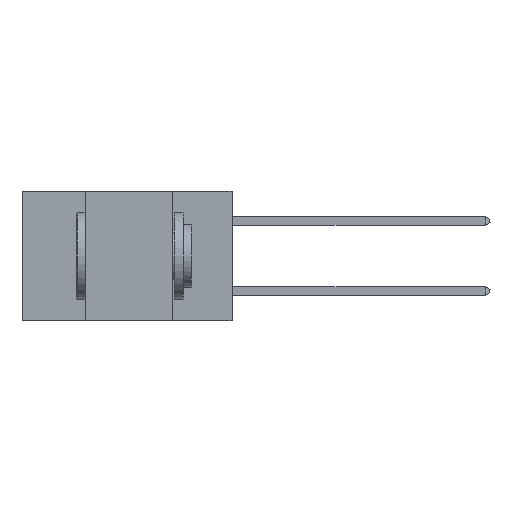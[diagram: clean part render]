
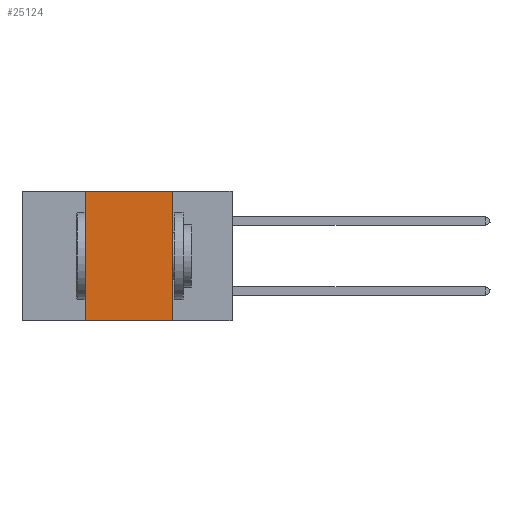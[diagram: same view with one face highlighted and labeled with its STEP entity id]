
A CAD part, left-side view. The second image highlights one B-rep face of the part: STEP entity #25124.
In plain terms, the highlighted planar face has unit normal (-1, 0, 0).
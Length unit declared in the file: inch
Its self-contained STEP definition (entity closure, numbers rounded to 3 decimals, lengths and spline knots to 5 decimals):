
#597 = CARTESIAN_POINT ( 'NONE',  ( 0., 0.42, -0.37 ) ) ;
#2726 = EDGE_CURVE ( 'NONE', #23165, #25789, #34216, .T. ) ;
#4073 = VERTEX_POINT ( 'NONE', #22299 ) ;
#4488 = CARTESIAN_POINT ( 'NONE',  ( 0., 0.6, 0. ) ) ;
#5153 = ORIENTED_EDGE ( 'NONE', *, *, #2726, .F. ) ;
#6057 = ORIENTED_EDGE ( 'NONE', *, *, #22233, .F. ) ;
#7336 = FACE_OUTER_BOUND ( 'NONE', #36327, .T. ) ;
#9321 = PLANE ( 'NONE',  #26371 ) ;
#10691 = VECTOR ( 'NONE', #11193, 39.37008 ) ;
#10835 = CARTESIAN_POINT ( 'NONE',  ( 0., 0.17, 0. ) ) ;
#11193 = DIRECTION ( 'NONE',  ( 0., 0., -1. ) ) ;
#12261 = CARTESIAN_POINT ( 'NONE',  ( 0., 0.17, -0.37 ) ) ;
#15567 = VECTOR ( 'NONE', #27453, 39.37008 ) ;
#17461 = VECTOR ( 'NONE', #36445, 39.37008 ) ;
#17555 = LINE ( 'NONE', #18975, #31771 ) ;
#17823 = DIRECTION ( 'NONE',  ( 1., 0., 0. ) ) ;
#18363 = LINE ( 'NONE', #33680, #17461 ) ;
#18975 = CARTESIAN_POINT ( 'NONE',  ( 0., 0.42, 0. ) ) ;
#21882 = DIRECTION ( 'NONE',  ( 0., 0., 1. ) ) ;
#22233 = EDGE_CURVE ( 'NONE', #34912, #4073, #17555, .T. ) ;
#22299 = CARTESIAN_POINT ( 'NONE',  ( 0., 0.42, 0. ) ) ;
#23165 = VERTEX_POINT ( 'NONE', #28659 ) ;
#23631 = CARTESIAN_POINT ( 'NONE',  ( 0., 0.6, 0. ) ) ;
#25124 = ADVANCED_FACE ( 'NONE', ( #7336 ), #9321, .F. ) ;
#25789 = VERTEX_POINT ( 'NONE', #12261 ) ;
#26371 = AXIS2_PLACEMENT_3D ( 'NONE', #23631, #17823, #29335 ) ;
#27453 = DIRECTION ( 'NONE',  ( 0., -1., 0. ) ) ;
#28048 = ORIENTED_EDGE ( 'NONE', *, *, #31682, .F. ) ;
#28659 = CARTESIAN_POINT ( 'NONE',  ( 0., 0.17, 0. ) ) ;
#29335 = DIRECTION ( 'NONE',  ( 0., 0., -1. ) ) ;
#30666 = ORIENTED_EDGE ( 'NONE', *, *, #36035, .T. ) ;
#31602 = LINE ( 'NONE', #4488, #15567 ) ;
#31682 = EDGE_CURVE ( 'NONE', #4073, #23165, #31602, .T. ) ;
#31771 = VECTOR ( 'NONE', #21882, 39.37008 ) ;
#33680 = CARTESIAN_POINT ( 'NONE',  ( 0., 0.6, -0.37 ) ) ;
#34216 = LINE ( 'NONE', #10835, #10691 ) ;
#34912 = VERTEX_POINT ( 'NONE', #597 ) ;
#36035 = EDGE_CURVE ( 'NONE', #34912, #25789, #18363, .T. ) ;
#36327 = EDGE_LOOP ( 'NONE', ( #5153, #28048, #6057, #30666 ) ) ;
#36445 = DIRECTION ( 'NONE',  ( 0., -1., 0. ) ) ;
